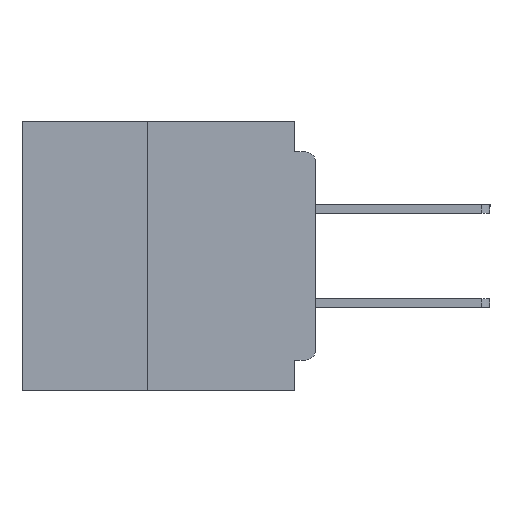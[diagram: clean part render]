
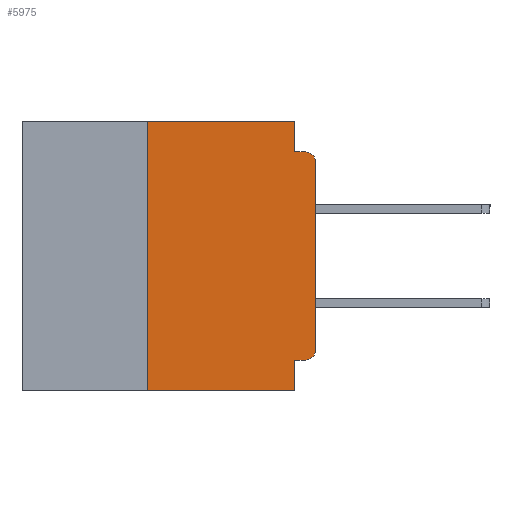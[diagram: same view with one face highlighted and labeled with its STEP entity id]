
A CAD part, left-side view. The second image highlights one B-rep face of the part: STEP entity #5975.
In plain terms, the highlighted planar face has unit normal (-1, 0, 0).
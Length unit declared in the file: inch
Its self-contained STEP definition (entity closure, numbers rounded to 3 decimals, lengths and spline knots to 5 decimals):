
#2538 = CARTESIAN_POINT ( 'NONE',  ( 0., 0.437, 0. ) ) ;
#3447 = VECTOR ( 'NONE', #53104, 39.37008 ) ;
#3536 = LINE ( 'NONE', #22594, #41007 ) ;
#3904 = DIRECTION ( 'NONE',  ( 0., 0., -1. ) ) ;
#4842 = ORIENTED_EDGE ( 'NONE', *, *, #39236, .F. ) ;
#5121 = ORIENTED_EDGE ( 'NONE', *, *, #52186, .F. ) ;
#5536 = DIRECTION ( 'NONE',  ( -1., 0., 0. ) ) ;
#5975 = ADVANCED_FACE ( 'NONE', ( #60188 ), #11859, .F. ) ;
#7477 = DIRECTION ( 'NONE',  ( 0., -1., 0. ) ) ;
#7855 = EDGE_CURVE ( 'NONE', #9771, #10630, #3536, .T. ) ;
#9251 = CARTESIAN_POINT ( 'NONE',  ( 0., 0.031, 0. ) ) ;
#9378 = VERTEX_POINT ( 'NONE', #9390 ) ;
#9390 = CARTESIAN_POINT ( 'NONE',  ( 0., 0.015, -0.355 ) ) ;
#9771 = VERTEX_POINT ( 'NONE', #12736 ) ;
#10447 = EDGE_CURVE ( 'NONE', #9771, #60928, #30244, .T. ) ;
#10630 = VERTEX_POINT ( 'NONE', #29836 ) ;
#10708 = VERTEX_POINT ( 'NONE', #44910 ) ;
#11112 = VECTOR ( 'NONE', #7477, 39.37008 ) ;
#11327 = CARTESIAN_POINT ( 'NONE',  ( 0., 0.031, -0.4 ) ) ;
#11614 = LINE ( 'NONE', #38955, #48999 ) ;
#11859 = PLANE ( 'NONE',  #26334 ) ;
#11883 = LINE ( 'NONE', #14280, #23402 ) ;
#11978 = CARTESIAN_POINT ( 'NONE',  ( 0., 0., 0. ) ) ;
#12736 = CARTESIAN_POINT ( 'NONE',  ( 0., 0.25, -0.4 ) ) ;
#13772 = VERTEX_POINT ( 'NONE', #19998 ) ;
#14280 = CARTESIAN_POINT ( 'NONE',  ( 0., 0.031, 0. ) ) ;
#16820 = ORIENTED_EDGE ( 'NONE', *, *, #10447, .T. ) ;
#16903 = LINE ( 'NONE', #11978, #44410 ) ;
#17037 = EDGE_CURVE ( 'NONE', #10708, #13772, #55329, .T. ) ;
#17176 = VECTOR ( 'NONE', #43025, 39.37008 ) ;
#19653 = VERTEX_POINT ( 'NONE', #40126 ) ;
#19998 = CARTESIAN_POINT ( 'NONE',  ( 0., 0.015, -0.045 ) ) ;
#20643 = VERTEX_POINT ( 'NONE', #9251 ) ;
#22594 = CARTESIAN_POINT ( 'NONE',  ( 0., 0.25, -0.4 ) ) ;
#23402 = VECTOR ( 'NONE', #43529, 39.37008 ) ;
#23622 = ORIENTED_EDGE ( 'NONE', *, *, #7855, .F. ) ;
#24769 = ORIENTED_EDGE ( 'NONE', *, *, #60330, .T. ) ;
#26334 = AXIS2_PLACEMENT_3D ( 'NONE', #26687, #60602, #31607 ) ;
#26484 = EDGE_CURVE ( 'NONE', #19653, #26535, #16903, .T. ) ;
#26535 = VERTEX_POINT ( 'NONE', #56102 ) ;
#26687 = CARTESIAN_POINT ( 'NONE',  ( 0., 0.437, 0. ) ) ;
#28826 = CARTESIAN_POINT ( 'NONE',  ( 0., 0.031, -0.4 ) ) ;
#29409 = ORIENTED_EDGE ( 'NONE', *, *, #26484, .T. ) ;
#29836 = CARTESIAN_POINT ( 'NONE',  ( 0., 0.25, 0. ) ) ;
#30244 = LINE ( 'NONE', #57399, #17176 ) ;
#31607 = DIRECTION ( 'NONE',  ( 0., 0., -1. ) ) ;
#32589 = ORIENTED_EDGE ( 'NONE', *, *, #45473, .T. ) ;
#33257 = DIRECTION ( 'NONE',  ( -1., 0., 0. ) ) ;
#33638 = CARTESIAN_POINT ( 'NONE',  ( 0., 0., -0.045 ) ) ;
#34282 = LINE ( 'NONE', #11327, #58512 ) ;
#34879 = CARTESIAN_POINT ( 'NONE',  ( 0., 0.015, -0.06 ) ) ;
#35661 = LINE ( 'NONE', #2538, #11112 ) ;
#38864 = VERTEX_POINT ( 'NONE', #62826 ) ;
#38955 = CARTESIAN_POINT ( 'NONE',  ( 0., 0., -0.355 ) ) ;
#39236 = EDGE_CURVE ( 'NONE', #10630, #20643, #35661, .T. ) ;
#39745 = DIRECTION ( 'NONE',  ( 0., 0., -1. ) ) ;
#40126 = CARTESIAN_POINT ( 'NONE',  ( 0., 0., -0.34 ) ) ;
#40993 = CIRCLE ( 'NONE', #60907, 0.015 ) ;
#41007 = VECTOR ( 'NONE', #56609, 39.37008 ) ;
#43025 = DIRECTION ( 'NONE',  ( 0., -1., 0. ) ) ;
#43529 = DIRECTION ( 'NONE',  ( 0., 0., -1. ) ) ;
#44198 = CIRCLE ( 'NONE', #51559, 0.015 ) ;
#44410 = VECTOR ( 'NONE', #50761, 39.37008 ) ;
#44910 = CARTESIAN_POINT ( 'NONE',  ( 0., 0.031, -0.045 ) ) ;
#45473 = EDGE_CURVE ( 'NONE', #9378, #19653, #44198, .T. ) ;
#45531 = DIRECTION ( 'NONE',  ( 0., 0., -1. ) ) ;
#45816 = EDGE_CURVE ( 'NONE', #38864, #60928, #34282, .T. ) ;
#47835 = EDGE_CURVE ( 'NONE', #9378, #38864, #11614, .T. ) ;
#48999 = VECTOR ( 'NONE', #63039, 39.37008 ) ;
#49493 = ORIENTED_EDGE ( 'NONE', *, *, #47835, .F. ) ;
#50761 = DIRECTION ( 'NONE',  ( 0., 0., 1. ) ) ;
#51559 = AXIS2_PLACEMENT_3D ( 'NONE', #62218, #33257, #3904 ) ;
#52186 = EDGE_CURVE ( 'NONE', #20643, #10708, #11883, .T. ) ;
#53104 = DIRECTION ( 'NONE',  ( 0., -1., 0. ) ) ;
#55329 = LINE ( 'NONE', #33638, #3447 ) ;
#56015 = ORIENTED_EDGE ( 'NONE', *, *, #45816, .F. ) ;
#56102 = CARTESIAN_POINT ( 'NONE',  ( 0., 0., -0.06 ) ) ;
#56259 = ORIENTED_EDGE ( 'NONE', *, *, #17037, .F. ) ;
#56609 = DIRECTION ( 'NONE',  ( 0., 0., 1. ) ) ;
#57399 = CARTESIAN_POINT ( 'NONE',  ( 0., 0.437, -0.4 ) ) ;
#58512 = VECTOR ( 'NONE', #45531, 39.37008 ) ;
#60188 = FACE_OUTER_BOUND ( 'NONE', #60395, .T. ) ;
#60330 = EDGE_CURVE ( 'NONE', #26535, #13772, #40993, .T. ) ;
#60395 = EDGE_LOOP ( 'NONE', ( #29409, #24769, #56259, #5121, #4842, #23622, #16820, #56015, #49493, #32589 ) ) ;
#60602 = DIRECTION ( 'NONE',  ( 1., 0., 0. ) ) ;
#60907 = AXIS2_PLACEMENT_3D ( 'NONE', #34879, #5536, #39745 ) ;
#60928 = VERTEX_POINT ( 'NONE', #28826 ) ;
#62218 = CARTESIAN_POINT ( 'NONE',  ( 0., 0.015, -0.34 ) ) ;
#62826 = CARTESIAN_POINT ( 'NONE',  ( 0., 0.031, -0.355 ) ) ;
#63039 = DIRECTION ( 'NONE',  ( 0., 1., 0. ) ) ;
